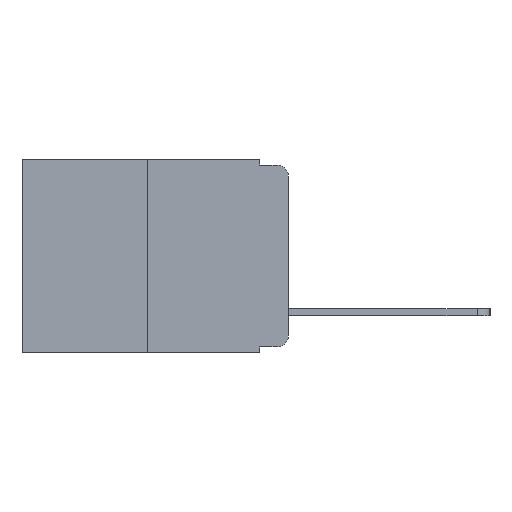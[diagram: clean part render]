
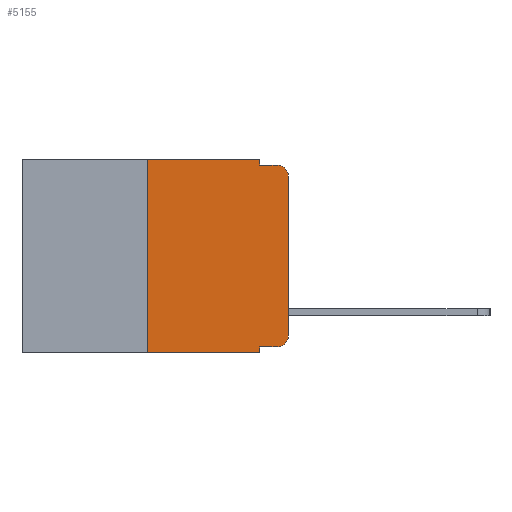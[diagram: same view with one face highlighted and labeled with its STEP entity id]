
A CAD part, left-side view. The second image highlights one B-rep face of the part: STEP entity #5155.
In plain terms, the highlighted planar face has unit normal (-1, 0, 0).
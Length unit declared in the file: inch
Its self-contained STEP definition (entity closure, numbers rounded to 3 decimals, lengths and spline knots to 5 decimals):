
#154 = CIRCLE ( 'NONE', #5827, 0.02 ) ;
#391 = DIRECTION ( 'NONE',  ( 0., -1., 0. ) ) ;
#483 = CARTESIAN_POINT ( 'NONE',  ( 0., 0.25, -0.343 ) ) ;
#765 = DIRECTION ( 'NONE',  ( 0., -1., 0. ) ) ;
#986 = VERTEX_POINT ( 'NONE', #16814 ) ;
#1003 = VERTEX_POINT ( 'NONE', #9716 ) ;
#1348 = ORIENTED_EDGE ( 'NONE', *, *, #13747, .F. ) ;
#1828 = DIRECTION ( 'NONE',  ( -1., 0., 0. ) ) ;
#1992 = VERTEX_POINT ( 'NONE', #483 ) ;
#2199 = VERTEX_POINT ( 'NONE', #6816 ) ;
#2399 = PLANE ( 'NONE',  #7565 ) ;
#2577 = DIRECTION ( 'NONE',  ( 0., 0., -1. ) ) ;
#3413 = VECTOR ( 'NONE', #16889, 39.37008 ) ;
#3595 = VERTEX_POINT ( 'NONE', #11976 ) ;
#3819 = VERTEX_POINT ( 'NONE', #7774 ) ;
#4421 = CARTESIAN_POINT ( 'NONE',  ( 0., 0.473, 0. ) ) ;
#4675 = CARTESIAN_POINT ( 'NONE',  ( 0., 0.473, -0.343 ) ) ;
#4992 = VECTOR ( 'NONE', #2577, 39.37008 ) ;
#5023 = VERTEX_POINT ( 'NONE', #9922 ) ;
#5122 = ORIENTED_EDGE ( 'NONE', *, *, #14837, .F. ) ;
#5155 = ADVANCED_FACE ( 'NONE', ( #11950 ), #2399, .F. ) ;
#5281 = EDGE_CURVE ( 'NONE', #1992, #1003, #18059, .T. ) ;
#5783 = LINE ( 'NONE', #15087, #13024 ) ;
#5827 = AXIS2_PLACEMENT_3D ( 'NONE', #15000, #6399, #16392 ) ;
#5872 = DIRECTION ( 'NONE',  ( 0., 0., -1. ) ) ;
#6399 = DIRECTION ( 'NONE',  ( -1., 0., 0. ) ) ;
#6489 = CARTESIAN_POINT ( 'NONE',  ( 0., 0.25, 0. ) ) ;
#6508 = ORIENTED_EDGE ( 'NONE', *, *, #11867, .F. ) ;
#6532 = VECTOR ( 'NONE', #12307, 39.37008 ) ;
#6662 = VECTOR ( 'NONE', #9075, 39.37008 ) ;
#6816 = CARTESIAN_POINT ( 'NONE',  ( 0., 0., -0.03 ) ) ;
#6827 = ORIENTED_EDGE ( 'NONE', *, *, #5281, .T. ) ;
#6842 = VECTOR ( 'NONE', #13660, 39.37008 ) ;
#7565 = AXIS2_PLACEMENT_3D ( 'NONE', #4421, #14520, #5872 ) ;
#7639 = EDGE_LOOP ( 'NONE', ( #9079, #18173, #1348, #6508, #5122, #10294, #6827, #12250, #15988, #15970 ) ) ;
#7643 = CARTESIAN_POINT ( 'NONE',  ( 0., 0.051, -0.01 ) ) ;
#7774 = CARTESIAN_POINT ( 'NONE',  ( 0., 0.02, -0.333 ) ) ;
#7969 = EDGE_CURVE ( 'NONE', #3819, #986, #154, .T. ) ;
#8668 = CIRCLE ( 'NONE', #13426, 0.02 ) ;
#8951 = EDGE_CURVE ( 'NONE', #5023, #3819, #10743, .T. ) ;
#9075 = DIRECTION ( 'NONE',  ( 0., -1., 0. ) ) ;
#9079 = ORIENTED_EDGE ( 'NONE', *, *, #15625, .T. ) ;
#9716 = CARTESIAN_POINT ( 'NONE',  ( 0., 0.051, -0.343 ) ) ;
#9922 = CARTESIAN_POINT ( 'NONE',  ( 0., 0.051, -0.333 ) ) ;
#9941 = EDGE_CURVE ( 'NONE', #5023, #1003, #12686, .T. ) ;
#10294 = ORIENTED_EDGE ( 'NONE', *, *, #10916, .F. ) ;
#10519 = CARTESIAN_POINT ( 'NONE',  ( 0., 0.02, -0.03 ) ) ;
#10615 = CARTESIAN_POINT ( 'NONE',  ( 0., 0.051, -0.333 ) ) ;
#10743 = LINE ( 'NONE', #10615, #14068 ) ;
#10916 = EDGE_CURVE ( 'NONE', #1992, #3595, #18373, .T. ) ;
#11027 = VERTEX_POINT ( 'NONE', #15376 ) ;
#11867 = EDGE_CURVE ( 'NONE', #18145, #14720, #5783, .T. ) ;
#11950 = FACE_OUTER_BOUND ( 'NONE', #7639, .T. ) ;
#11951 = DIRECTION ( 'NONE',  ( 0., 0., -1. ) ) ;
#11976 = CARTESIAN_POINT ( 'NONE',  ( 0., 0.25, 0. ) ) ;
#12250 = ORIENTED_EDGE ( 'NONE', *, *, #9941, .F. ) ;
#12307 = DIRECTION ( 'NONE',  ( 0., 0., 1. ) ) ;
#12686 = LINE ( 'NONE', #18340, #4992 ) ;
#13024 = VECTOR ( 'NONE', #16481, 39.37008 ) ;
#13426 = AXIS2_PLACEMENT_3D ( 'NONE', #10519, #1828, #11951 ) ;
#13660 = DIRECTION ( 'NONE',  ( 0., -1., 0. ) ) ;
#13747 = EDGE_CURVE ( 'NONE', #14720, #11027, #18042, .T. ) ;
#13885 = CARTESIAN_POINT ( 'NONE',  ( 0., 0.051, 0. ) ) ;
#14017 = LINE ( 'NONE', #18317, #3413 ) ;
#14057 = LINE ( 'NONE', #16470, #6842 ) ;
#14068 = VECTOR ( 'NONE', #391, 39.37008 ) ;
#14335 = VECTOR ( 'NONE', #765, 39.37008 ) ;
#14520 = DIRECTION ( 'NONE',  ( 1., 0., 0. ) ) ;
#14701 = EDGE_CURVE ( 'NONE', #2199, #11027, #8668, .T. ) ;
#14720 = VERTEX_POINT ( 'NONE', #7643 ) ;
#14837 = EDGE_CURVE ( 'NONE', #3595, #18145, #14057, .T. ) ;
#15000 = CARTESIAN_POINT ( 'NONE',  ( 0., 0.02, -0.313 ) ) ;
#15087 = CARTESIAN_POINT ( 'NONE',  ( 0., 0.051, 0. ) ) ;
#15376 = CARTESIAN_POINT ( 'NONE',  ( 0., 0.02, -0.01 ) ) ;
#15625 = EDGE_CURVE ( 'NONE', #986, #2199, #14017, .T. ) ;
#15970 = ORIENTED_EDGE ( 'NONE', *, *, #7969, .T. ) ;
#15988 = ORIENTED_EDGE ( 'NONE', *, *, #8951, .T. ) ;
#16392 = DIRECTION ( 'NONE',  ( 0., 0., -1. ) ) ;
#16470 = CARTESIAN_POINT ( 'NONE',  ( 0., 0.473, 0. ) ) ;
#16481 = DIRECTION ( 'NONE',  ( 0., 0., -1. ) ) ;
#16531 = CARTESIAN_POINT ( 'NONE',  ( 0., 0.051, -0.01 ) ) ;
#16814 = CARTESIAN_POINT ( 'NONE',  ( 0., 0., -0.313 ) ) ;
#16889 = DIRECTION ( 'NONE',  ( 0., 0., 1. ) ) ;
#18042 = LINE ( 'NONE', #16531, #14335 ) ;
#18059 = LINE ( 'NONE', #4675, #6662 ) ;
#18145 = VERTEX_POINT ( 'NONE', #13885 ) ;
#18173 = ORIENTED_EDGE ( 'NONE', *, *, #14701, .T. ) ;
#18317 = CARTESIAN_POINT ( 'NONE',  ( 0., 0., 0. ) ) ;
#18340 = CARTESIAN_POINT ( 'NONE',  ( 0., 0.051, 0. ) ) ;
#18373 = LINE ( 'NONE', #6489, #6532 ) ;
